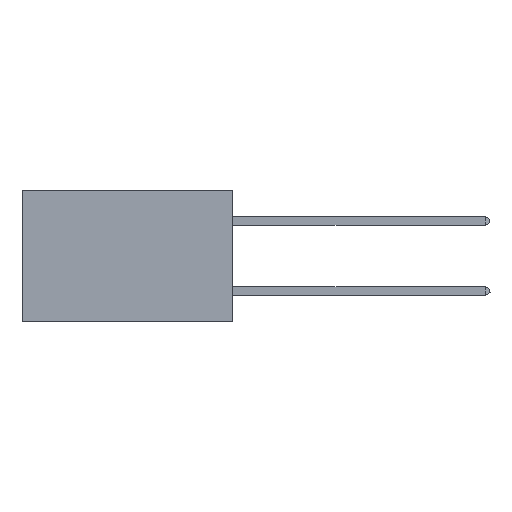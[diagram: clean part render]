
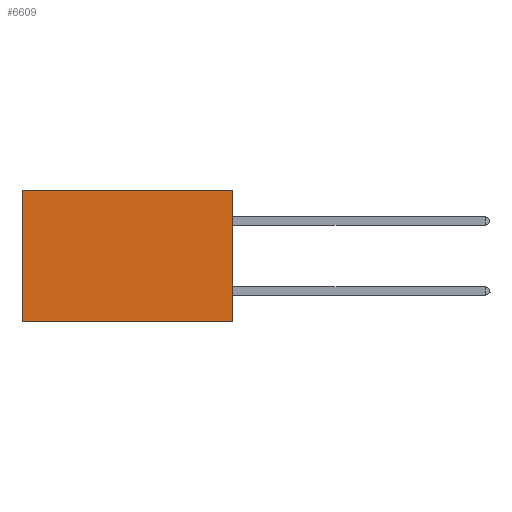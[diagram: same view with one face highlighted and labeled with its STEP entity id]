
A CAD part, left-side view. The second image highlights one B-rep face of the part: STEP entity #6609.
In plain terms, the highlighted planar face has unit normal (-1, 0, 0).
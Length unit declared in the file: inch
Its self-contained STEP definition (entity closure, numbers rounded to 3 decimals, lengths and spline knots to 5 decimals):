
#244 = VECTOR ( 'NONE', #16556, 39.37008 ) ;
#1294 = VERTEX_POINT ( 'NONE', #5445 ) ;
#1325 = VECTOR ( 'NONE', #14266, 39.37008 ) ;
#1422 = ORIENTED_EDGE ( 'NONE', *, *, #10750, .F. ) ;
#2232 = ORIENTED_EDGE ( 'NONE', *, *, #4967, .T. ) ;
#3228 = EDGE_CURVE ( 'NONE', #15453, #8075, #5727, .T. ) ;
#4795 = DIRECTION ( 'NONE',  ( 1., 0., 0. ) ) ;
#4938 = DIRECTION ( 'NONE',  ( 0., 0., -1. ) ) ;
#4967 = EDGE_CURVE ( 'NONE', #5394, #15453, #19394, .T. ) ;
#5088 = EDGE_CURVE ( 'NONE', #5394, #1294, #18356, .T. ) ;
#5387 = CARTESIAN_POINT ( 'NONE',  ( 0.2875, 0.6, 0. ) ) ;
#5394 = VERTEX_POINT ( 'NONE', #15781 ) ;
#5445 = CARTESIAN_POINT ( 'NONE',  ( 0.2875, 0., -0.375 ) ) ;
#5727 = LINE ( 'NONE', #9605, #1325 ) ;
#6609 = ADVANCED_FACE ( 'NONE', ( #6644 ), #14909, .F. ) ;
#6644 = FACE_OUTER_BOUND ( 'NONE', #18041, .T. ) ;
#6829 = CARTESIAN_POINT ( 'NONE',  ( 0.2875, 0., -0.375 ) ) ;
#6943 = DIRECTION ( 'NONE',  ( 0., 0., -1. ) ) ;
#8075 = VERTEX_POINT ( 'NONE', #20030 ) ;
#8775 = VECTOR ( 'NONE', #19842, 39.37008 ) ;
#9605 = CARTESIAN_POINT ( 'NONE',  ( 0.2875, 0.6, -0.375 ) ) ;
#9676 = CARTESIAN_POINT ( 'NONE',  ( 0.2875, 0., -0.375 ) ) ;
#9846 = AXIS2_PLACEMENT_3D ( 'NONE', #9676, #4795, #4938 ) ;
#10085 = LINE ( 'NONE', #6829, #244 ) ;
#10750 = EDGE_CURVE ( 'NONE', #1294, #8075, #10085, .T. ) ;
#11349 = ORIENTED_EDGE ( 'NONE', *, *, #5088, .F. ) ;
#12681 = VECTOR ( 'NONE', #6943, 39.37008 ) ;
#13188 = CARTESIAN_POINT ( 'NONE',  ( 0.2875, 0., 0. ) ) ;
#14266 = DIRECTION ( 'NONE',  ( 0., 0., -1. ) ) ;
#14500 = ORIENTED_EDGE ( 'NONE', *, *, #3228, .T. ) ;
#14909 = PLANE ( 'NONE',  #9846 ) ;
#15453 = VERTEX_POINT ( 'NONE', #5387 ) ;
#15781 = CARTESIAN_POINT ( 'NONE',  ( 0.2875, 0., 0. ) ) ;
#16556 = DIRECTION ( 'NONE',  ( 0., 1., 0. ) ) ;
#18041 = EDGE_LOOP ( 'NONE', ( #14500, #1422, #11349, #2232 ) ) ;
#18356 = LINE ( 'NONE', #20119, #12681 ) ;
#19394 = LINE ( 'NONE', #13188, #8775 ) ;
#19842 = DIRECTION ( 'NONE',  ( 0., 1., 0. ) ) ;
#20030 = CARTESIAN_POINT ( 'NONE',  ( 0.2875, 0.6, -0.375 ) ) ;
#20119 = CARTESIAN_POINT ( 'NONE',  ( 0.2875, 0., -0.375 ) ) ;
